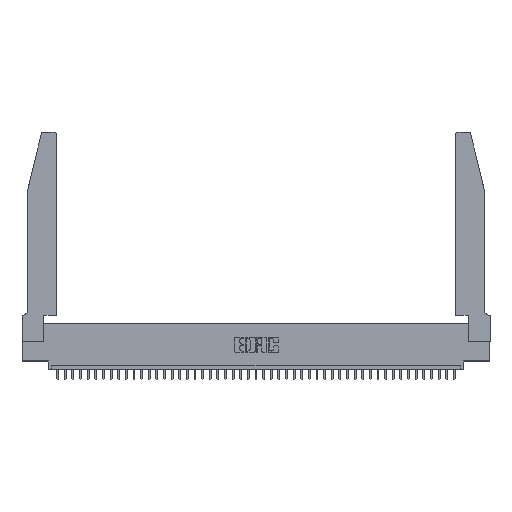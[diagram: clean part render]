
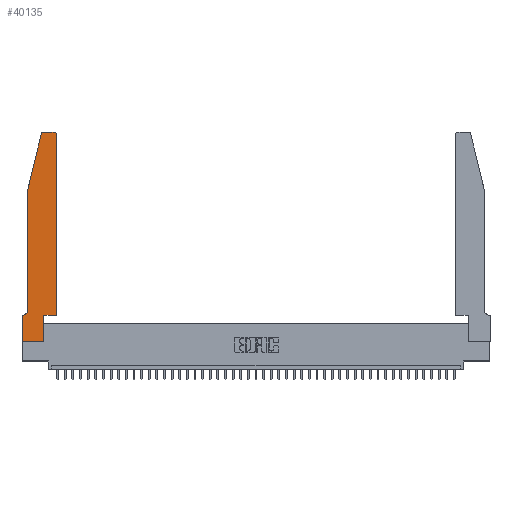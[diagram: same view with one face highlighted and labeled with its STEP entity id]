
A CAD part, top view. The second image highlights one B-rep face of the part: STEP entity #40135.
In plain terms, the highlighted planar face has unit normal (0, 0, 1).
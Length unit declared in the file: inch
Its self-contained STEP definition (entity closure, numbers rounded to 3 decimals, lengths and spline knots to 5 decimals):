
#494 = CARTESIAN_POINT ( 'NONE',  ( 0.2865, 0.35, 0.37 ) ) ;
#582 = DIRECTION ( 'NONE',  ( 0., 0., 1. ) ) ;
#933 = CARTESIAN_POINT ( 'NONE',  ( 0.0755, 0.35, 0.37 ) ) ;
#1607 = ORIENTED_EDGE ( 'NONE', *, *, #21210, .T. ) ;
#2044 = LINE ( 'NONE', #10654, #36537 ) ;
#2269 = ORIENTED_EDGE ( 'NONE', *, *, #12261, .T. ) ;
#2837 = DIRECTION ( 'NONE',  ( -1., 0., 0. ) ) ;
#3091 = EDGE_CURVE ( 'NONE', #6378, #4565, #3936, .T. ) ;
#3295 = LINE ( 'NONE', #933, #13804 ) ;
#3936 = LINE ( 'NONE', #37020, #42139 ) ;
#3963 = VERTEX_POINT ( 'NONE', #39358 ) ;
#4153 = LINE ( 'NONE', #38862, #28242 ) ;
#4565 = VERTEX_POINT ( 'NONE', #36101 ) ;
#4909 = DIRECTION ( 'NONE',  ( -1., 0., 0. ) ) ;
#5093 = CARTESIAN_POINT ( 'NONE',  ( 0., 0.35, 0.37 ) ) ;
#5805 = AXIS2_PLACEMENT_3D ( 'NONE', #20191, #37499, #10538 ) ;
#5965 = FACE_OUTER_BOUND ( 'NONE', #26101, .T. ) ;
#6378 = VERTEX_POINT ( 'NONE', #41093 ) ;
#6682 = DIRECTION ( 'NONE',  ( 1., 0., 0. ) ) ;
#7656 = LINE ( 'NONE', #11043, #35332 ) ;
#8172 = VERTEX_POINT ( 'NONE', #40631 ) ;
#8364 = DIRECTION ( 'NONE',  ( 0., 1., 0. ) ) ;
#8711 = AXIS2_PLACEMENT_3D ( 'NONE', #40644, #582, #36949 ) ;
#9275 = CIRCLE ( 'NONE', #8711, 0.03 ) ;
#9793 = VERTEX_POINT ( 'NONE', #18007 ) ;
#10167 = AXIS2_PLACEMENT_3D ( 'NONE', #28160, #23674, #2837 ) ;
#10185 = DIRECTION ( 'NONE',  ( 0., 1., 0. ) ) ;
#10538 = DIRECTION ( 'NONE',  ( 1., 0., 0. ) ) ;
#10573 = ORIENTED_EDGE ( 'NONE', *, *, #32123, .T. ) ;
#10654 = CARTESIAN_POINT ( 'NONE',  ( 0.0755, 2., 0.37 ) ) ;
#10927 = CARTESIAN_POINT ( 'NONE',  ( 0.2605, 2.75, 0.37 ) ) ;
#11043 = CARTESIAN_POINT ( 'NONE',  ( 0.0755, 2., 0.37 ) ) ;
#11045 = CARTESIAN_POINT ( 'NONE',  ( 0.4505, 0.35, 0.37 ) ) ;
#11156 = LINE ( 'NONE', #34663, #23199 ) ;
#11925 = PLANE ( 'NONE',  #35984 ) ;
#12200 = VERTEX_POINT ( 'NONE', #40342 ) ;
#12261 = EDGE_CURVE ( 'NONE', #12200, #29061, #3295, .T. ) ;
#12277 = EDGE_CURVE ( 'NONE', #39629, #36685, #11156, .T. ) ;
#13763 = VERTEX_POINT ( 'NONE', #39148 ) ;
#13804 = VECTOR ( 'NONE', #4909, 39.37008 ) ;
#14028 = DIRECTION ( 'NONE',  ( 0., -1., 0. ) ) ;
#14396 = DIRECTION ( 'NONE',  ( -0.239, -0.971, 0. ) ) ;
#15579 = ORIENTED_EDGE ( 'NONE', *, *, #18764, .T. ) ;
#15818 = EDGE_CURVE ( 'NONE', #13763, #9793, #7656, .T. ) ;
#15871 = CARTESIAN_POINT ( 'NONE',  ( 0., 0.35, 0.37 ) ) ;
#16448 = DIRECTION ( 'NONE',  ( 0., 0., 1. ) ) ;
#17830 = LINE ( 'NONE', #36299, #27745 ) ;
#18007 = CARTESIAN_POINT ( 'NONE',  ( 0.0755, 2., 0.37 ) ) ;
#18020 = VERTEX_POINT ( 'NONE', #40776 ) ;
#18165 = ORIENTED_EDGE ( 'NONE', *, *, #40799, .T. ) ;
#18764 = EDGE_CURVE ( 'NONE', #36685, #3963, #17830, .T. ) ;
#19079 = EDGE_CURVE ( 'NONE', #4565, #39629, #4153, .T. ) ;
#20191 = CARTESIAN_POINT ( 'NONE',  ( 0.4205, 2.72, 0.37 ) ) ;
#21210 = EDGE_CURVE ( 'NONE', #8172, #18020, #32174, .T. ) ;
#21340 = ORIENTED_EDGE ( 'NONE', *, *, #26600, .T. ) ;
#21521 = CIRCLE ( 'NONE', #5805, 0.03 ) ;
#22179 = DIRECTION ( 'NONE',  ( 1., 0., 0. ) ) ;
#23012 = DIRECTION ( 'NONE',  ( 1., 0., 0. ) ) ;
#23199 = VECTOR ( 'NONE', #22179, 39.37008 ) ;
#23631 = EDGE_CURVE ( 'NONE', #18020, #13763, #9275, .T. ) ;
#23674 = DIRECTION ( 'NONE',  ( 0., 0., -1. ) ) ;
#25552 = ORIENTED_EDGE ( 'NONE', *, *, #23631, .T. ) ;
#26101 = EDGE_LOOP ( 'NONE', ( #1607, #25552, #29632, #30188, #21340, #2269, #18165, #32529, #39045, #42637, #15579, #10573 ) ) ;
#26600 = EDGE_CURVE ( 'NONE', #29611, #12200, #40928, .T. ) ;
#27745 = VECTOR ( 'NONE', #10185, 39.37008 ) ;
#28108 = EDGE_CURVE ( 'NONE', #9793, #29611, #2044, .T. ) ;
#28160 = CARTESIAN_POINT ( 'NONE',  ( 0.0055, 0.42, 0.37 ) ) ;
#28242 = VECTOR ( 'NONE', #8364, 39.37008 ) ;
#28433 = CARTESIAN_POINT ( 'NONE',  ( 0.0755, 0.42, 0.37 ) ) ;
#28904 = VECTOR ( 'NONE', #14028, 39.37008 ) ;
#29061 = VERTEX_POINT ( 'NONE', #5093 ) ;
#29611 = VERTEX_POINT ( 'NONE', #28433 ) ;
#29632 = ORIENTED_EDGE ( 'NONE', *, *, #15818, .T. ) ;
#30188 = ORIENTED_EDGE ( 'NONE', *, *, #28108, .T. ) ;
#30964 = LINE ( 'NONE', #33979, #28904 ) ;
#31033 = DIRECTION ( 'NONE',  ( -1., 0., 0. ) ) ;
#32123 = EDGE_CURVE ( 'NONE', #3963, #8172, #21521, .T. ) ;
#32174 = LINE ( 'NONE', #10927, #33197 ) ;
#32529 = ORIENTED_EDGE ( 'NONE', *, *, #3091, .T. ) ;
#33197 = VECTOR ( 'NONE', #31033, 39.37008 ) ;
#33836 = DIRECTION ( 'NONE',  ( 0., -1., 0. ) ) ;
#33979 = CARTESIAN_POINT ( 'NONE',  ( 0., 0., 0.37 ) ) ;
#34663 = CARTESIAN_POINT ( 'NONE',  ( 0.4505, 0.35, 0.37 ) ) ;
#35332 = VECTOR ( 'NONE', #14396, 39.37008 ) ;
#35984 = AXIS2_PLACEMENT_3D ( 'NONE', #15871, #16448, #23012 ) ;
#36101 = CARTESIAN_POINT ( 'NONE',  ( 0.2865, 0., 0.37 ) ) ;
#36299 = CARTESIAN_POINT ( 'NONE',  ( 0.4505, 0.35, 0.37 ) ) ;
#36537 = VECTOR ( 'NONE', #33836, 39.37008 ) ;
#36685 = VERTEX_POINT ( 'NONE', #11045 ) ;
#36949 = DIRECTION ( 'NONE',  ( 1., 0., 0. ) ) ;
#37020 = CARTESIAN_POINT ( 'NONE',  ( 0., 0., 0.37 ) ) ;
#37499 = DIRECTION ( 'NONE',  ( 0., 0., 1. ) ) ;
#38862 = CARTESIAN_POINT ( 'NONE',  ( 0.2865, 0.35, 0.37 ) ) ;
#39045 = ORIENTED_EDGE ( 'NONE', *, *, #19079, .T. ) ;
#39148 = CARTESIAN_POINT ( 'NONE',  ( 0.25487, 2.72718, 0.37 ) ) ;
#39358 = CARTESIAN_POINT ( 'NONE',  ( 0.4505, 2.72, 0.37 ) ) ;
#39629 = VERTEX_POINT ( 'NONE', #494 ) ;
#40135 = ADVANCED_FACE ( 'NONE', ( #5965 ), #11925, .T. ) ;
#40342 = CARTESIAN_POINT ( 'NONE',  ( 0.0055, 0.35, 0.37 ) ) ;
#40631 = CARTESIAN_POINT ( 'NONE',  ( 0.4205, 2.75, 0.37 ) ) ;
#40644 = CARTESIAN_POINT ( 'NONE',  ( 0.284, 2.72, 0.37 ) ) ;
#40776 = CARTESIAN_POINT ( 'NONE',  ( 0.284, 2.75, 0.37 ) ) ;
#40799 = EDGE_CURVE ( 'NONE', #29061, #6378, #30964, .T. ) ;
#40928 = CIRCLE ( 'NONE', #10167, 0.07 ) ;
#41093 = CARTESIAN_POINT ( 'NONE',  ( 0., 0., 0.37 ) ) ;
#42139 = VECTOR ( 'NONE', #6682, 39.37008 ) ;
#42637 = ORIENTED_EDGE ( 'NONE', *, *, #12277, .T. ) ;
